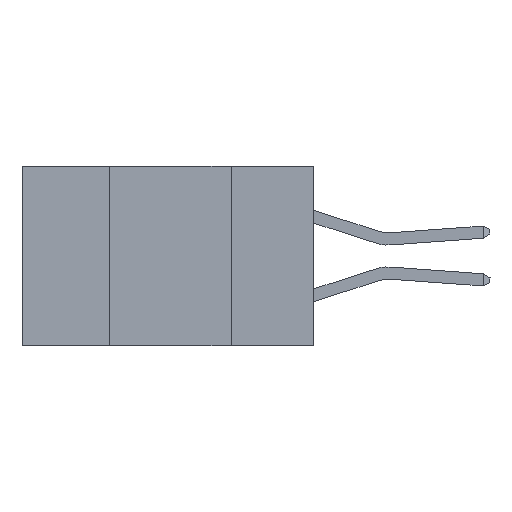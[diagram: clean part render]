
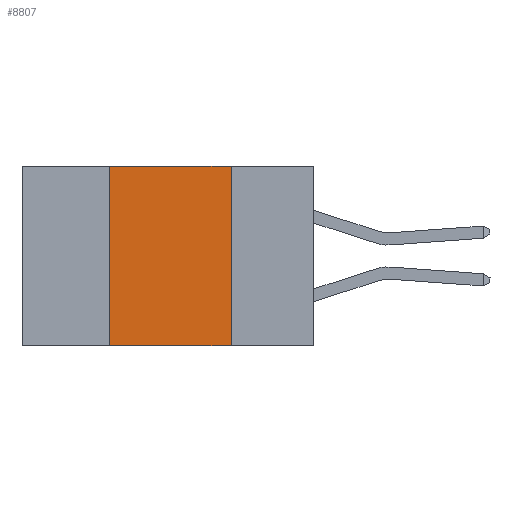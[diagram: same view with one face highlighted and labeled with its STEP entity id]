
A CAD part, left-side view. The second image highlights one B-rep face of the part: STEP entity #8807.
In plain terms, the highlighted planar face has unit normal (-1, 0, 0).
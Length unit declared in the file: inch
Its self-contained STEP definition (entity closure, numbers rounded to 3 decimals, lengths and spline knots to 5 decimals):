
#912 = VERTEX_POINT ( 'NONE', #7301 ) ;
#1176 = CARTESIAN_POINT ( 'NONE',  ( 0., 0.17, 0. ) ) ;
#1563 = ORIENTED_EDGE ( 'NONE', *, *, #7408, .F. ) ;
#1771 = LINE ( 'NONE', #8041, #5775 ) ;
#1853 = LINE ( 'NONE', #9770, #9979 ) ;
#1957 = EDGE_CURVE ( 'NONE', #2971, #912, #7543, .T. ) ;
#2285 = CARTESIAN_POINT ( 'NONE',  ( 0., 0.17, -0.37 ) ) ;
#2729 = CARTESIAN_POINT ( 'NONE',  ( 0., 0.6, 0. ) ) ;
#2971 = VERTEX_POINT ( 'NONE', #7344 ) ;
#3540 = DIRECTION ( 'NONE',  ( 0., 0., -1. ) ) ;
#3581 = DIRECTION ( 'NONE',  ( 0., 0., 1. ) ) ;
#3594 = DIRECTION ( 'NONE',  ( 0., -1., 0. ) ) ;
#4313 = VERTEX_POINT ( 'NONE', #1176 ) ;
#4663 = EDGE_CURVE ( 'NONE', #4313, #5829, #1771, .T. ) ;
#4842 = EDGE_CURVE ( 'NONE', #2971, #5829, #8021, .T. ) ;
#5144 = DIRECTION ( 'NONE',  ( 0., -1., 0. ) ) ;
#5408 = VECTOR ( 'NONE', #3581, 39.37008 ) ;
#5775 = VECTOR ( 'NONE', #7236, 39.37008 ) ;
#5819 = ORIENTED_EDGE ( 'NONE', *, *, #1957, .F. ) ;
#5829 = VERTEX_POINT ( 'NONE', #2285 ) ;
#5894 = VECTOR ( 'NONE', #5144, 39.37008 ) ;
#6262 = EDGE_LOOP ( 'NONE', ( #7711, #1563, #5819, #7953 ) ) ;
#6944 = FACE_OUTER_BOUND ( 'NONE', #6262, .T. ) ;
#7236 = DIRECTION ( 'NONE',  ( 0., 0., -1. ) ) ;
#7301 = CARTESIAN_POINT ( 'NONE',  ( 0., 0.42, 0. ) ) ;
#7344 = CARTESIAN_POINT ( 'NONE',  ( 0., 0.42, -0.37 ) ) ;
#7408 = EDGE_CURVE ( 'NONE', #912, #4313, #1853, .T. ) ;
#7480 = PLANE ( 'NONE',  #10062 ) ;
#7521 = CARTESIAN_POINT ( 'NONE',  ( 0., 0.6, -0.37 ) ) ;
#7543 = LINE ( 'NONE', #7606, #5408 ) ;
#7606 = CARTESIAN_POINT ( 'NONE',  ( 0., 0.42, 0. ) ) ;
#7711 = ORIENTED_EDGE ( 'NONE', *, *, #4663, .F. ) ;
#7953 = ORIENTED_EDGE ( 'NONE', *, *, #4842, .T. ) ;
#8021 = LINE ( 'NONE', #7521, #5894 ) ;
#8041 = CARTESIAN_POINT ( 'NONE',  ( 0., 0.17, 0. ) ) ;
#8246 = DIRECTION ( 'NONE',  ( 1., 0., 0. ) ) ;
#8807 = ADVANCED_FACE ( 'NONE', ( #6944 ), #7480, .F. ) ;
#9770 = CARTESIAN_POINT ( 'NONE',  ( 0., 0.6, 0. ) ) ;
#9979 = VECTOR ( 'NONE', #3594, 39.37008 ) ;
#10062 = AXIS2_PLACEMENT_3D ( 'NONE', #2729, #8246, #3540 ) ;
